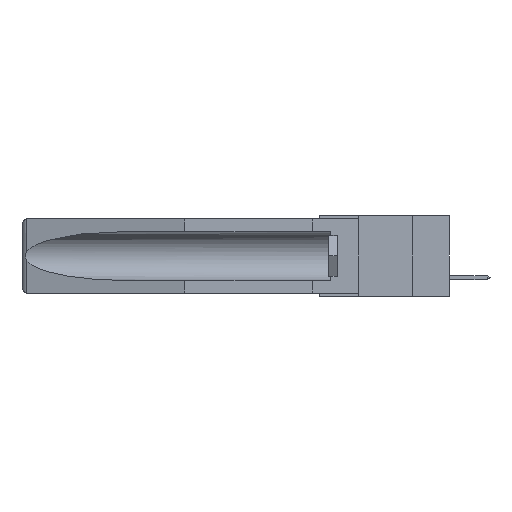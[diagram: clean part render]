
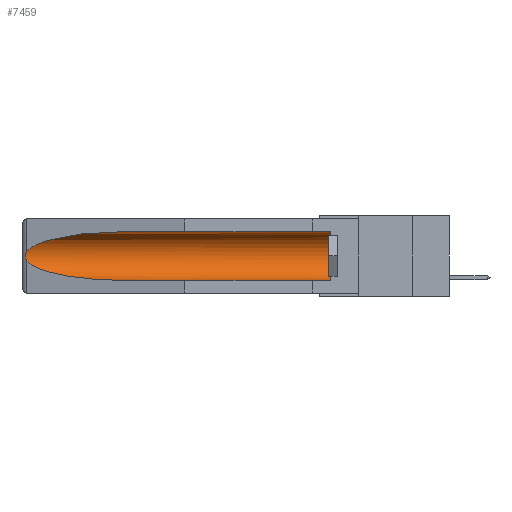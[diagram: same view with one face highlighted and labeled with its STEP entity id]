
A CAD part, left-side view. The second image highlights one B-rep face of the part: STEP entity #7459.
In plain terms, the highlighted cylindrical face has radius 2.857 mm (diameter 5.715 mm), a partial arc.
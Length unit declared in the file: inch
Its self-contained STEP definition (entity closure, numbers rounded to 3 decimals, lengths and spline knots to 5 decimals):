
#341 = VERTEX_POINT ( 'NONE', #11836 ) ;
#458 = CARTESIAN_POINT ( 'NONE',  ( 0.155, 0.126, -0.059 ) ) ;
#521 = ORIENTED_EDGE ( 'NONE', *, *, #16833, .T. ) ;
#621 = ORIENTED_EDGE ( 'NONE', *, *, #8230, .T. ) ;
#832 = CARTESIAN_POINT ( 'NONE',  ( 0.26597, 1.52961, -0.15275 ) ) ;
#903 = CARTESIAN_POINT ( 'NONE',  ( 0.2673, 1.5327, -0.16383 ) ) ;
#1039 = VERTEX_POINT ( 'NONE', #4817 ) ;
#1181 = ORIENTED_EDGE ( 'NONE', *, *, #19240, .F. ) ;
#1338 = DIRECTION ( 'NONE',  ( 0., 0., 1. ) ) ;
#1412 = CARTESIAN_POINT ( 'NONE',  ( 0.26537, 1.52718, -0.14972 ) ) ;
#1485 = FACE_OUTER_BOUND ( 'NONE', #18220, .T. ) ;
#1529 =( BOUNDED_CURVE ( )  B_SPLINE_CURVE ( 3, ( #15116, #9018, #13439, #1412 ),
 .UNSPECIFIED., .F., .F. ) 
 B_SPLINE_CURVE_WITH_KNOTS ( ( 4, 4 ),
 ( 4.71239, 6.08839 ),
 .UNSPECIFIED. ) 
 CURVE ( )  GEOMETRIC_REPRESENTATION_ITEM ( )  RATIONAL_B_SPLINE_CURVE ( ( 1., 0.848, 0.848, 1. ) ) 
 REPRESENTATION_ITEM ( '' )  );
#2121 = EDGE_CURVE ( 'NONE', #1039, #15078, #8838, .T. ) ;
#2354 =( BOUNDED_CURVE ( )  B_SPLINE_CURVE ( 3, ( #12629, #10975, #9432, #11043 ),
 .UNSPECIFIED., .F., .F. ) 
 B_SPLINE_CURVE_WITH_KNOTS ( ( 4, 4 ),
 ( 0.1948, 1.5708 ),
 .UNSPECIFIED. ) 
 CURVE ( )  GEOMETRIC_REPRESENTATION_ITEM ( )  RATIONAL_B_SPLINE_CURVE ( ( 1., 0.848, 0.848, 1. ) ) 
 REPRESENTATION_ITEM ( '' )  );
#2515 = CARTESIAN_POINT ( 'NONE',  ( 0.26537, 1.52718, -0.14972 ) ) ;
#3659 = VERTEX_POINT ( 'NONE', #6527 ) ;
#3761 = EDGE_CURVE ( 'NONE', #3659, #341, #17063, .T. ) ;
#3946 = CARTESIAN_POINT ( 'NONE',  ( 0.26654, 1.53092, -0.15636 ) ) ;
#4300 = AXIS2_PLACEMENT_3D ( 'NONE', #13899, #9208, #15173 ) ;
#4319 = DIRECTION ( 'NONE',  ( 0., -1., 0. ) ) ;
#4510 = LINE ( 'NONE', #14779, #17928 ) ;
#4817 = CARTESIAN_POINT ( 'NONE',  ( 0.155, 0.126, -0.284 ) ) ;
#5571 = VECTOR ( 'NONE', #9186, 39.37008 ) ;
#5864 = ORIENTED_EDGE ( 'NONE', *, *, #3761, .T. ) ;
#6525 = VERTEX_POINT ( 'NONE', #19075 ) ;
#6527 = CARTESIAN_POINT ( 'NONE',  ( 0.26537, 1.52718, -0.14972 ) ) ;
#7047 = CARTESIAN_POINT ( 'NONE',  ( 0.2673, 1.53269, -0.17917 ) ) ;
#7459 = ADVANCED_FACE ( 'NONE', ( #1485 ), #17745, .F. ) ;
#7460 = AXIS2_PLACEMENT_3D ( 'NONE', #13763, #4319, #1338 ) ;
#8230 = EDGE_CURVE ( 'NONE', #14119, #3659, #1529, .T. ) ;
#8838 = CIRCLE ( 'NONE', #7460, 0.1125 ) ;
#8915 = CARTESIAN_POINT ( 'NONE',  ( 0.26597, 1.5296, -0.19026 ) ) ;
#9018 = CARTESIAN_POINT ( 'NONE',  ( 0.21114, 1.30732, -0.059 ) ) ;
#9186 = DIRECTION ( 'NONE',  ( 0., 1., 0. ) ) ;
#9208 = DIRECTION ( 'NONE',  ( 0., 1., 0. ) ) ;
#9432 = CARTESIAN_POINT ( 'NONE',  ( 0.21114, 1.30732, -0.284 ) ) ;
#10214 = DIRECTION ( 'NONE',  ( 0., 1., 0. ) ) ;
#10975 = CARTESIAN_POINT ( 'NONE',  ( 0.25451, 1.48313, -0.24835 ) ) ;
#11043 = CARTESIAN_POINT ( 'NONE',  ( 0.155, 1.07973, -0.284 ) ) ;
#11165 = EDGE_CURVE ( 'NONE', #15078, #14119, #18296, .T. ) ;
#11603 = CARTESIAN_POINT ( 'NONE',  ( 0.2675, 1.53308, -0.16763 ) ) ;
#11836 = CARTESIAN_POINT ( 'NONE',  ( 0.26537, 1.52718, -0.19328 ) ) ;
#12096 = ORIENTED_EDGE ( 'NONE', *, *, #11165, .T. ) ;
#12629 = CARTESIAN_POINT ( 'NONE',  ( 0.26537, 1.52718, -0.19328 ) ) ;
#13136 = CARTESIAN_POINT ( 'NONE',  ( 0.2675, 1.53308, -0.17534 ) ) ;
#13439 = CARTESIAN_POINT ( 'NONE',  ( 0.25451, 1.48313, -0.09465 ) ) ;
#13763 = CARTESIAN_POINT ( 'NONE',  ( 0.155, 0.126, -0.1715 ) ) ;
#13899 = CARTESIAN_POINT ( 'NONE',  ( 0.155, -0.30754, -0.1715 ) ) ;
#14119 = VERTEX_POINT ( 'NONE', #16456 ) ;
#14779 = CARTESIAN_POINT ( 'NONE',  ( 0.155, -0.30754, -0.284 ) ) ;
#15078 = VERTEX_POINT ( 'NONE', #458 ) ;
#15116 = CARTESIAN_POINT ( 'NONE',  ( 0.155, 1.07973, -0.059 ) ) ;
#15173 = DIRECTION ( 'NONE',  ( 0., 0., 1. ) ) ;
#15229 = CARTESIAN_POINT ( 'NONE',  ( 0.155, -0.30754, -0.059 ) ) ;
#15933 = ORIENTED_EDGE ( 'NONE', *, *, #2121, .T. ) ;
#16448 = CARTESIAN_POINT ( 'NONE',  ( 0.26655, 1.53094, -0.18657 ) ) ;
#16456 = CARTESIAN_POINT ( 'NONE',  ( 0.155, 1.07973, -0.059 ) ) ;
#16504 = CARTESIAN_POINT ( 'NONE',  ( 0.26537, 1.52718, -0.19328 ) ) ;
#16833 = EDGE_CURVE ( 'NONE', #341, #6525, #2354, .T. ) ;
#17063 = B_SPLINE_CURVE_WITH_KNOTS ( 'NONE', 3,
 ( #2515, #832, #3946, #903, #11603, #13136, #7047, #16448, #8915, #16504 ),
 .UNSPECIFIED., .F., .F.,
 ( 4, 2, 2, 2, 4 ),
 ( 0., 0.00029, 0.00058, 0.00087, 0.00117 ),
 .UNSPECIFIED. ) ;
#17745 = CYLINDRICAL_SURFACE ( 'NONE', #4300, 0.1125 ) ;
#17928 = VECTOR ( 'NONE', #10214, 39.37008 ) ;
#18220 = EDGE_LOOP ( 'NONE', ( #621, #5864, #521, #1181, #15933, #12096 ) ) ;
#18296 = LINE ( 'NONE', #15229, #5571 ) ;
#19075 = CARTESIAN_POINT ( 'NONE',  ( 0.155, 1.07973, -0.284 ) ) ;
#19240 = EDGE_CURVE ( 'NONE', #1039, #6525, #4510, .T. ) ;
